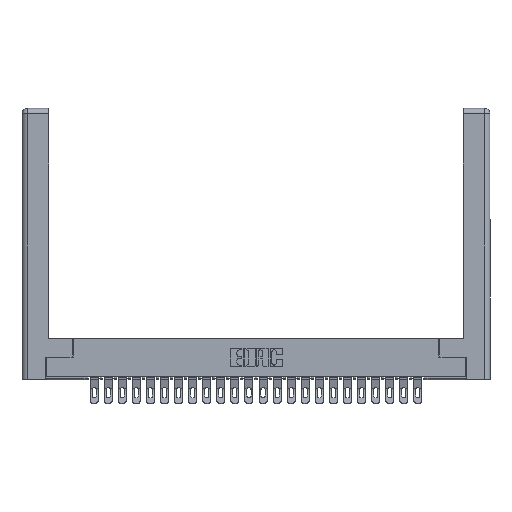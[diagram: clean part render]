
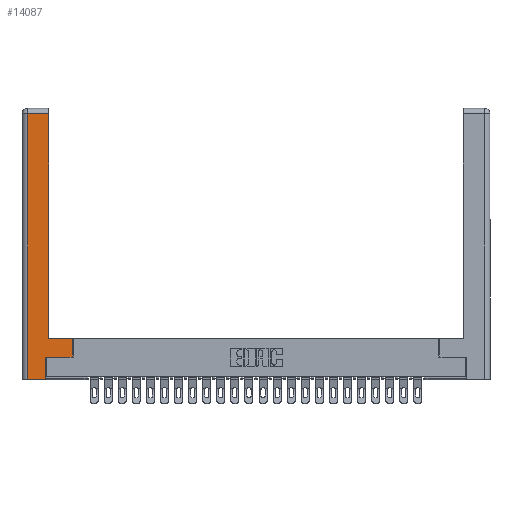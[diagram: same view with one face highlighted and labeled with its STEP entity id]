
A CAD part, top view. The second image highlights one B-rep face of the part: STEP entity #14087.
In plain terms, the highlighted planar face has unit normal (0, 0, 1).
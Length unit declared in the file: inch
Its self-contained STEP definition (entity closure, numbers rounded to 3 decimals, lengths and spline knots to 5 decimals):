
#140 = VECTOR ( 'NONE', #29383, 39.37008 ) ;
#393 = CARTESIAN_POINT ( 'NONE',  ( 0., 0., 0. ) ) ;
#596 = ORIENTED_EDGE ( 'NONE', *, *, #10274, .T. ) ;
#607 = CARTESIAN_POINT ( 'NONE',  ( 0.565, 0.45, 0. ) ) ;
#737 = CARTESIAN_POINT ( 'NONE',  ( 0.265, 0.245, 0. ) ) ;
#770 = EDGE_CURVE ( 'NONE', #25797, #5148, #16529, .T. ) ;
#965 = ORIENTED_EDGE ( 'NONE', *, *, #6353, .T. ) ;
#1071 = DIRECTION ( 'NONE',  ( -1., 0., 0. ) ) ;
#1196 = DIRECTION ( 'NONE',  ( 0., -1., 0. ) ) ;
#1230 = EDGE_CURVE ( 'NONE', #17738, #18149, #14235, .T. ) ;
#1509 = VECTOR ( 'NONE', #27169, 39.37008 ) ;
#2412 = VECTOR ( 'NONE', #15438, 39.37008 ) ;
#2758 = CARTESIAN_POINT ( 'NONE',  ( 0.265, 0., 0. ) ) ;
#2802 = LINE ( 'NONE', #6100, #16536 ) ;
#2895 = EDGE_LOOP ( 'NONE', ( #13159, #19939, #596, #9779, #965, #6769, #21642, #23962 ) ) ;
#3408 = CARTESIAN_POINT ( 'NONE',  ( 0.565, 0.245, 0. ) ) ;
#3843 = EDGE_CURVE ( 'NONE', #30187, #17738, #9323, .T. ) ;
#3848 = EDGE_CURVE ( 'NONE', #18149, #25797, #2802, .T. ) ;
#4558 = DIRECTION ( 'NONE',  ( -1., 0., 0. ) ) ;
#4582 = LINE ( 'NONE', #2758, #1509 ) ;
#4900 = VECTOR ( 'NONE', #4558, 39.37008 ) ;
#5148 = VERTEX_POINT ( 'NONE', #16999 ) ;
#5633 = CARTESIAN_POINT ( 'NONE',  ( 0.565, 0.245, 0. ) ) ;
#6100 = CARTESIAN_POINT ( 'NONE',  ( 0.295, 0.45, 0. ) ) ;
#6353 = EDGE_CURVE ( 'NONE', #12107, #30187, #6551, .T. ) ;
#6551 = LINE ( 'NONE', #737, #17167 ) ;
#6769 = ORIENTED_EDGE ( 'NONE', *, *, #3843, .T. ) ;
#7019 = CARTESIAN_POINT ( 'NONE',  ( 0.0615, 2.94, 0. ) ) ;
#7121 = VECTOR ( 'NONE', #1196, 39.37008 ) ;
#7128 = VERTEX_POINT ( 'NONE', #8511 ) ;
#7642 = PLANE ( 'NONE',  #8730 ) ;
#7663 = CARTESIAN_POINT ( 'NONE',  ( 0.295, 0.45, 0. ) ) ;
#8212 = DIRECTION ( 'NONE',  ( 0., 1., 0. ) ) ;
#8511 = CARTESIAN_POINT ( 'NONE',  ( 0.0615, 0., 0. ) ) ;
#8730 = AXIS2_PLACEMENT_3D ( 'NONE', #393, #14683, #24711 ) ;
#9047 = DIRECTION ( 'NONE',  ( 0., 1., 0. ) ) ;
#9323 = LINE ( 'NONE', #3408, #2412 ) ;
#9779 = ORIENTED_EDGE ( 'NONE', *, *, #14719, .T. ) ;
#10274 = EDGE_CURVE ( 'NONE', #14665, #7128, #26851, .T. ) ;
#11374 = LINE ( 'NONE', #7019, #4900 ) ;
#12107 = VERTEX_POINT ( 'NONE', #31196 ) ;
#13159 = ORIENTED_EDGE ( 'NONE', *, *, #770, .T. ) ;
#14087 = ADVANCED_FACE ( 'NONE', ( #27759 ), #7642, .F. ) ;
#14235 = LINE ( 'NONE', #607, #140 ) ;
#14440 = CARTESIAN_POINT ( 'NONE',  ( 0.565, 0.45, 0. ) ) ;
#14665 = VERTEX_POINT ( 'NONE', #17035 ) ;
#14683 = DIRECTION ( 'NONE',  ( 0., 0., -1. ) ) ;
#14719 = EDGE_CURVE ( 'NONE', #7128, #12107, #4582, .T. ) ;
#15438 = DIRECTION ( 'NONE',  ( 1., 0., 0. ) ) ;
#16529 = LINE ( 'NONE', #16684, #23734 ) ;
#16536 = VECTOR ( 'NONE', #1071, 39.37008 ) ;
#16684 = CARTESIAN_POINT ( 'NONE',  ( 0.295, 3., 0. ) ) ;
#16999 = CARTESIAN_POINT ( 'NONE',  ( 0.295, 2.94, 0. ) ) ;
#17035 = CARTESIAN_POINT ( 'NONE',  ( 0.0615, 2.94, 0. ) ) ;
#17167 = VECTOR ( 'NONE', #8212, 39.37008 ) ;
#17213 = CARTESIAN_POINT ( 'NONE',  ( 0.265, 0.245, 0. ) ) ;
#17738 = VERTEX_POINT ( 'NONE', #5633 ) ;
#18020 = CARTESIAN_POINT ( 'NONE',  ( 0.0615, 0., 0. ) ) ;
#18149 = VERTEX_POINT ( 'NONE', #14440 ) ;
#19939 = ORIENTED_EDGE ( 'NONE', *, *, #26364, .T. ) ;
#21642 = ORIENTED_EDGE ( 'NONE', *, *, #1230, .T. ) ;
#23734 = VECTOR ( 'NONE', #9047, 39.37008 ) ;
#23962 = ORIENTED_EDGE ( 'NONE', *, *, #3848, .T. ) ;
#24711 = DIRECTION ( 'NONE',  ( -1., 0., 0. ) ) ;
#25797 = VERTEX_POINT ( 'NONE', #7663 ) ;
#26364 = EDGE_CURVE ( 'NONE', #5148, #14665, #11374, .T. ) ;
#26851 = LINE ( 'NONE', #18020, #7121 ) ;
#27169 = DIRECTION ( 'NONE',  ( 1., 0., 0. ) ) ;
#27759 = FACE_OUTER_BOUND ( 'NONE', #2895, .T. ) ;
#29383 = DIRECTION ( 'NONE',  ( 0., 1., 0. ) ) ;
#30187 = VERTEX_POINT ( 'NONE', #17213 ) ;
#31196 = CARTESIAN_POINT ( 'NONE',  ( 0.265, 0., 0. ) ) ;
